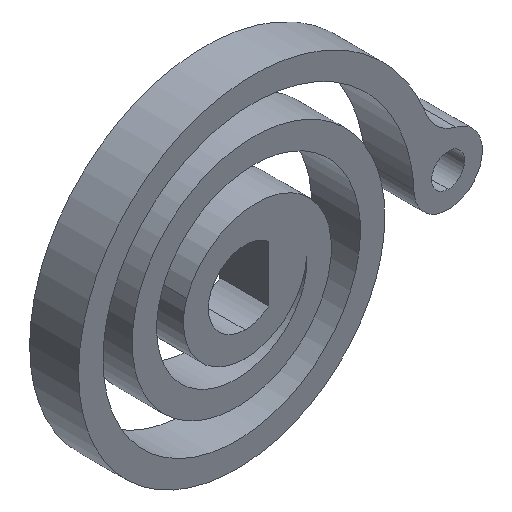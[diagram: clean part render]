
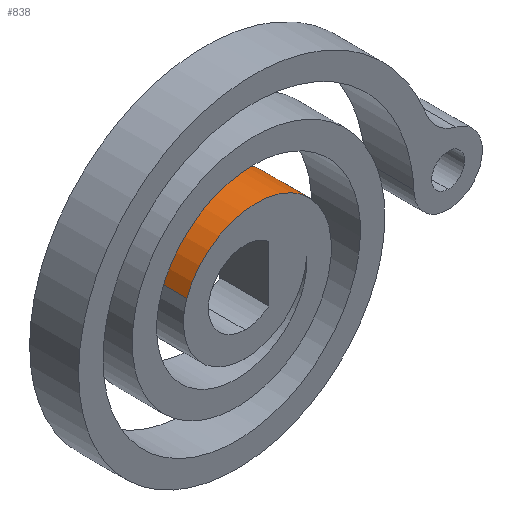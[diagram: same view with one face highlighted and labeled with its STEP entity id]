
A CAD part, isometric view. The second image highlights one B-rep face of the part: STEP entity #838.
In plain terms, the highlighted cylindrical face has radius 7.772 mm (diameter 15.545 mm), a partial arc.
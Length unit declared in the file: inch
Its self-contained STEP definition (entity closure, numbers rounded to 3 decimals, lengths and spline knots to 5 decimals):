
#16 = DIRECTION ( 'NONE',  ( 0., 1., 0. ) ) ;
#35 = CARTESIAN_POINT ( 'NONE',  ( 0.3515, 0., -0.00939 ) ) ;
#47 = DIRECTION ( 'NONE',  ( 0., 0., 1. ) ) ;
#113 = VERTEX_POINT ( 'NONE', #552 ) ;
#121 = AXIS2_PLACEMENT_3D ( 'NONE', #981, #495, #47 ) ;
#136 = FACE_OUTER_BOUND ( 'NONE', #313, .T. ) ;
#192 = DIRECTION ( 'NONE',  ( 0., -1., 0. ) ) ;
#271 = ORIENTED_EDGE ( 'NONE', *, *, #545, .T. ) ;
#288 = VERTEX_POINT ( 'NONE', #35 ) ;
#300 = ORIENTED_EDGE ( 'NONE', *, *, #493, .T. ) ;
#313 = EDGE_LOOP ( 'NONE', ( #271, #341, #439, #300 ) ) ;
#335 = VECTOR ( 'NONE', #192, 39.37008 ) ;
#341 = ORIENTED_EDGE ( 'NONE', *, *, #515, .F. ) ;
#399 = CARTESIAN_POINT ( 'NONE',  ( -0.23895, 0.2, 0.08102 ) ) ;
#404 = CYLINDRICAL_SURFACE ( 'NONE', #840, 0.30599 ) ;
#439 = ORIENTED_EDGE ( 'NONE', *, *, #672, .F. ) ;
#458 = CARTESIAN_POINT ( 'NONE',  ( 0.0462, 0., -0.03 ) ) ;
#493 = EDGE_CURVE ( 'NONE', #941, #992, #625, .T. ) ;
#495 = DIRECTION ( 'NONE',  ( 0., 1., 0. ) ) ;
#497 = CARTESIAN_POINT ( 'NONE',  ( 0.3515, 0.2, -0.00939 ) ) ;
#515 = EDGE_CURVE ( 'NONE', #113, #288, #949, .T. ) ;
#539 = AXIS2_PLACEMENT_3D ( 'NONE', #458, #16, #550 ) ;
#545 = EDGE_CURVE ( 'NONE', #992, #288, #822, .T. ) ;
#548 = DIRECTION ( 'NONE',  ( 0., -1., 0. ) ) ;
#550 = DIRECTION ( 'NONE',  ( 0., 0., 1. ) ) ;
#552 = CARTESIAN_POINT ( 'NONE',  ( 0.3515, 0.2, -0.00939 ) ) ;
#590 = DIRECTION ( 'NONE',  ( 0., -1., 0. ) ) ;
#612 = CARTESIAN_POINT ( 'NONE',  ( 0.0462, 0.2, -0.03 ) ) ;
#625 = LINE ( 'NONE', #399, #335 ) ;
#657 = CIRCLE ( 'NONE', #121, 0.30599 ) ;
#672 = EDGE_CURVE ( 'NONE', #941, #113, #657, .T. ) ;
#707 = DIRECTION ( 'NONE',  ( 0., 0., -1. ) ) ;
#709 = CARTESIAN_POINT ( 'NONE',  ( -0.23895, 0.2, 0.08102 ) ) ;
#822 = CIRCLE ( 'NONE', #539, 0.30599 ) ;
#838 = ADVANCED_FACE ( 'NONE', ( #136 ), #404, .T. ) ;
#839 = VECTOR ( 'NONE', #590, 39.37008 ) ;
#840 = AXIS2_PLACEMENT_3D ( 'NONE', #612, #548, #707 ) ;
#869 = CARTESIAN_POINT ( 'NONE',  ( -0.23895, 0., 0.08102 ) ) ;
#941 = VERTEX_POINT ( 'NONE', #709 ) ;
#949 = LINE ( 'NONE', #497, #839 ) ;
#981 = CARTESIAN_POINT ( 'NONE',  ( 0.0462, 0.2, -0.03 ) ) ;
#992 = VERTEX_POINT ( 'NONE', #869 ) ;
